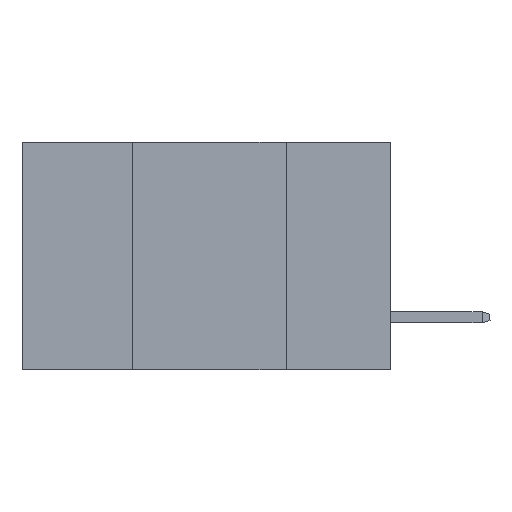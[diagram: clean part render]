
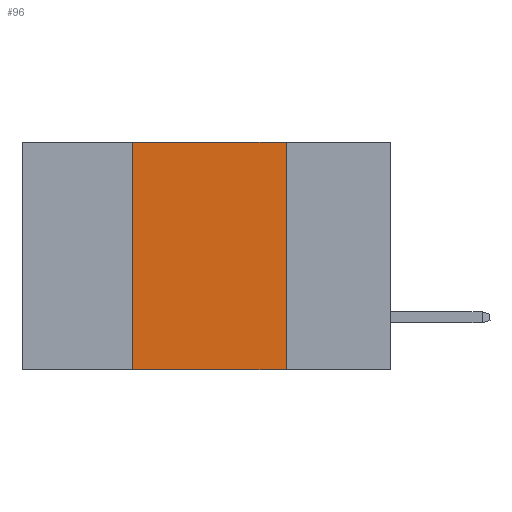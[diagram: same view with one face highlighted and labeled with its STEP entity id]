
A CAD part, left-side view. The second image highlights one B-rep face of the part: STEP entity #96.
In plain terms, the highlighted planar face has unit normal (-1, 0, 0).
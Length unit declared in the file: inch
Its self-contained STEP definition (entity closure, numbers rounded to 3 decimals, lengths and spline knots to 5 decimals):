
#96 = ADVANCED_FACE ( 'NONE', ( #5734 ), #1396, .F. ) ;
#458 = CARTESIAN_POINT ( 'NONE',  ( 0., 0.17, 0. ) ) ;
#750 = CARTESIAN_POINT ( 'NONE',  ( 0., 0.6, 0. ) ) ;
#1023 = CARTESIAN_POINT ( 'NONE',  ( 0., 0.42, -0.37 ) ) ;
#1349 = DIRECTION ( 'NONE',  ( 0., 0., -1. ) ) ;
#1396 = PLANE ( 'NONE',  #6776 ) ;
#1420 = EDGE_CURVE ( 'NONE', #3647, #6692, #8234, .T. ) ;
#1432 = ORIENTED_EDGE ( 'NONE', *, *, #7597, .F. ) ;
#1670 = CARTESIAN_POINT ( 'NONE',  ( 0., 0.17, -0.37 ) ) ;
#1675 = CARTESIAN_POINT ( 'NONE',  ( 0., 0.6, -0.37 ) ) ;
#1714 = DIRECTION ( 'NONE',  ( 0., -1., 0. ) ) ;
#2331 = VECTOR ( 'NONE', #6796, 39.37008 ) ;
#2747 = EDGE_LOOP ( 'NONE', ( #7532, #5150, #1432, #6362 ) ) ;
#3647 = VERTEX_POINT ( 'NONE', #1023 ) ;
#4251 = VECTOR ( 'NONE', #7634, 39.37008 ) ;
#4798 = DIRECTION ( 'NONE',  ( 1., 0., 0. ) ) ;
#4944 = CARTESIAN_POINT ( 'NONE',  ( 0., 0.17, 0. ) ) ;
#5150 = ORIENTED_EDGE ( 'NONE', *, *, #7692, .F. ) ;
#5227 = VERTEX_POINT ( 'NONE', #9275 ) ;
#5734 = FACE_OUTER_BOUND ( 'NONE', #2747, .T. ) ;
#5863 = LINE ( 'NONE', #6888, #4251 ) ;
#6362 = ORIENTED_EDGE ( 'NONE', *, *, #1420, .T. ) ;
#6692 = VERTEX_POINT ( 'NONE', #1670 ) ;
#6776 = AXIS2_PLACEMENT_3D ( 'NONE', #750, #4798, #1349 ) ;
#6796 = DIRECTION ( 'NONE',  ( 0., 0., 1. ) ) ;
#6888 = CARTESIAN_POINT ( 'NONE',  ( 0., 0.6, 0. ) ) ;
#6983 = EDGE_CURVE ( 'NONE', #9314, #6692, #8382, .T. ) ;
#7286 = VECTOR ( 'NONE', #9514, 39.37008 ) ;
#7532 = ORIENTED_EDGE ( 'NONE', *, *, #6983, .F. ) ;
#7597 = EDGE_CURVE ( 'NONE', #3647, #5227, #8475, .T. ) ;
#7634 = DIRECTION ( 'NONE',  ( 0., -1., 0. ) ) ;
#7692 = EDGE_CURVE ( 'NONE', #5227, #9314, #5863, .T. ) ;
#8228 = CARTESIAN_POINT ( 'NONE',  ( 0., 0.42, 0. ) ) ;
#8234 = LINE ( 'NONE', #1675, #8436 ) ;
#8382 = LINE ( 'NONE', #458, #7286 ) ;
#8436 = VECTOR ( 'NONE', #1714, 39.37008 ) ;
#8475 = LINE ( 'NONE', #8228, #2331 ) ;
#9275 = CARTESIAN_POINT ( 'NONE',  ( 0., 0.42, 0. ) ) ;
#9314 = VERTEX_POINT ( 'NONE', #4944 ) ;
#9514 = DIRECTION ( 'NONE',  ( 0., 0., -1. ) ) ;
